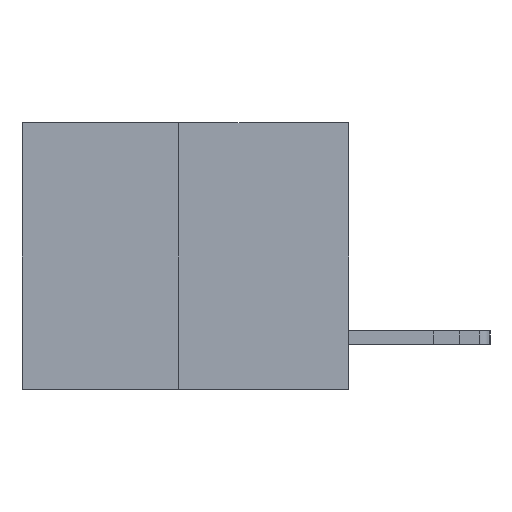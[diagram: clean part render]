
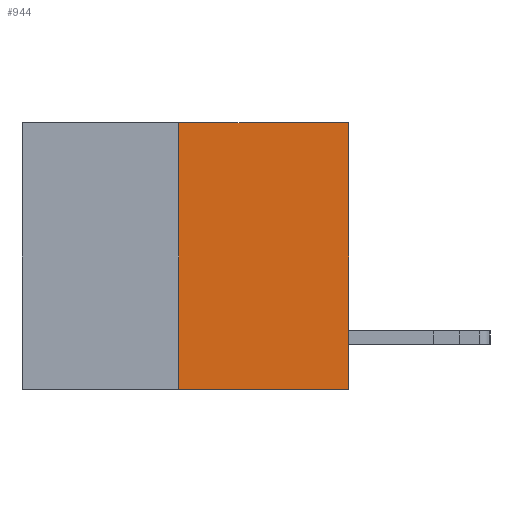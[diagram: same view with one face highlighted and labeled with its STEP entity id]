
A CAD part, left-side view. The second image highlights one B-rep face of the part: STEP entity #944.
In plain terms, the highlighted planar face has unit normal (-1, 0, 0).
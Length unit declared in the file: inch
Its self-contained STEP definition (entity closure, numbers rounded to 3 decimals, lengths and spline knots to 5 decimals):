
#555 = DIRECTION ( 'NONE',  ( 0., 0., -1. ) ) ;
#584 = CARTESIAN_POINT ( 'NONE',  ( 0., 0.312, -0.49 ) ) ;
#865 = ORIENTED_EDGE ( 'NONE', *, *, #10159, .F. ) ;
#944 = ADVANCED_FACE ( 'NONE', ( #9532 ), #14841, .F. ) ;
#1196 = EDGE_LOOP ( 'NONE', ( #1751, #6194, #8418, #865 ) ) ;
#1608 = LINE ( 'NONE', #2975, #8328 ) ;
#1751 = ORIENTED_EDGE ( 'NONE', *, *, #6035, .F. ) ;
#2832 = LINE ( 'NONE', #5969, #14308 ) ;
#2975 = CARTESIAN_POINT ( 'NONE',  ( 0., 0., 0. ) ) ;
#3845 = CARTESIAN_POINT ( 'NONE',  ( 0., 0., 0. ) ) ;
#4856 = CARTESIAN_POINT ( 'NONE',  ( 0., 0., -0.49 ) ) ;
#5395 = VERTEX_POINT ( 'NONE', #4856 ) ;
#5687 = DIRECTION ( 'NONE',  ( 0., -1., 0. ) ) ;
#5969 = CARTESIAN_POINT ( 'NONE',  ( 0., 0.312, -0.49 ) ) ;
#6035 = EDGE_CURVE ( 'NONE', #11748, #16876, #2832, .T. ) ;
#6194 = ORIENTED_EDGE ( 'NONE', *, *, #9495, .T. ) ;
#6468 = DIRECTION ( 'NONE',  ( 0., -1., 0. ) ) ;
#7298 = DIRECTION ( 'NONE',  ( 0., 0., 1. ) ) ;
#8328 = VECTOR ( 'NONE', #7298, 39.37008 ) ;
#8418 = ORIENTED_EDGE ( 'NONE', *, *, #16357, .T. ) ;
#9143 = VERTEX_POINT ( 'NONE', #3845 ) ;
#9232 = CARTESIAN_POINT ( 'NONE',  ( 0., 0.6, 0. ) ) ;
#9254 = LINE ( 'NONE', #9274, #12854 ) ;
#9274 = CARTESIAN_POINT ( 'NONE',  ( 0., 0.6, -0.49 ) ) ;
#9495 = EDGE_CURVE ( 'NONE', #11748, #5395, #9254, .T. ) ;
#9532 = FACE_OUTER_BOUND ( 'NONE', #1196, .T. ) ;
#10077 = CARTESIAN_POINT ( 'NONE',  ( 0., 0.6, 0. ) ) ;
#10159 = EDGE_CURVE ( 'NONE', #16876, #9143, #14858, .T. ) ;
#11748 = VERTEX_POINT ( 'NONE', #584 ) ;
#12854 = VECTOR ( 'NONE', #6468, 39.37008 ) ;
#14308 = VECTOR ( 'NONE', #16023, 39.37008 ) ;
#14497 = AXIS2_PLACEMENT_3D ( 'NONE', #9232, #14910, #555 ) ;
#14841 = PLANE ( 'NONE',  #14497 ) ;
#14858 = LINE ( 'NONE', #10077, #16212 ) ;
#14910 = DIRECTION ( 'NONE',  ( 1., 0., 0. ) ) ;
#16023 = DIRECTION ( 'NONE',  ( 0., 0., 1. ) ) ;
#16212 = VECTOR ( 'NONE', #5687, 39.37008 ) ;
#16357 = EDGE_CURVE ( 'NONE', #5395, #9143, #1608, .T. ) ;
#16876 = VERTEX_POINT ( 'NONE', #17066 ) ;
#17066 = CARTESIAN_POINT ( 'NONE',  ( 0., 0.312, 0. ) ) ;
